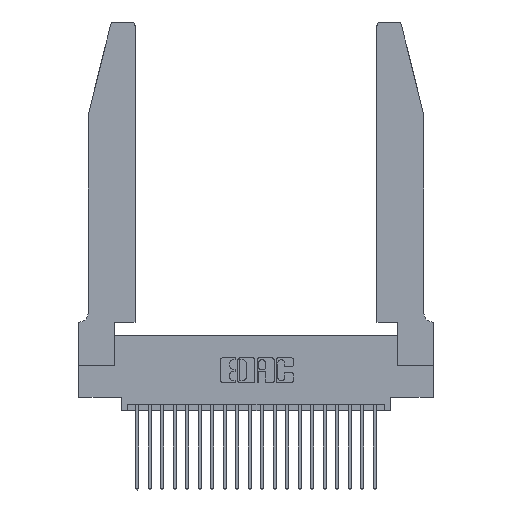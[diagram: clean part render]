
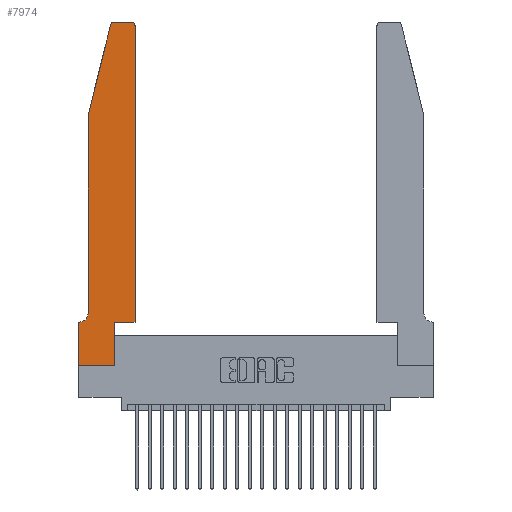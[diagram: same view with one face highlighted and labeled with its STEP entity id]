
A CAD part, top view. The second image highlights one B-rep face of the part: STEP entity #7974.
In plain terms, the highlighted planar face has unit normal (0, 0, 1).
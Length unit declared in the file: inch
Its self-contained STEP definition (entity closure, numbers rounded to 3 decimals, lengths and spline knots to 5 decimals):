
#375 = DIRECTION ( 'NONE',  ( 1., 0., 0. ) ) ;
#386 = EDGE_CURVE ( 'NONE', #14922, #15033, #14284, .T. ) ;
#395 = FACE_OUTER_BOUND ( 'NONE', #5012, .T. ) ;
#712 = DIRECTION ( 'NONE',  ( -1., 0., 0. ) ) ;
#841 = ORIENTED_EDGE ( 'NONE', *, *, #11650, .T. ) ;
#1287 = DIRECTION ( 'NONE',  ( 0., 0., 1. ) ) ;
#1448 = EDGE_CURVE ( 'NONE', #20195, #18270, #11090, .T. ) ;
#1613 = VECTOR ( 'NONE', #18647, 39.37008 ) ;
#2149 = DIRECTION ( 'NONE',  ( -0.239, -0.971, 0. ) ) ;
#2186 = VERTEX_POINT ( 'NONE', #14202 ) ;
#2226 = CARTESIAN_POINT ( 'NONE',  ( 0., 0., 0.37 ) ) ;
#2346 = DIRECTION ( 'NONE',  ( 1., 0., 0. ) ) ;
#2390 = CARTESIAN_POINT ( 'NONE',  ( 0.2865, 0.35, 0.37 ) ) ;
#2464 = EDGE_CURVE ( 'NONE', #11010, #21786, #21974, .T. ) ;
#2804 = CARTESIAN_POINT ( 'NONE',  ( 0., 0., 0.37 ) ) ;
#2820 = CARTESIAN_POINT ( 'NONE',  ( 0.4205, 2.72, 0.37 ) ) ;
#2937 = ORIENTED_EDGE ( 'NONE', *, *, #9304, .T. ) ;
#3006 = CARTESIAN_POINT ( 'NONE',  ( 0.4205, 2.75, 0.37 ) ) ;
#3283 = VECTOR ( 'NONE', #2346, 39.37008 ) ;
#4457 = DIRECTION ( 'NONE',  ( 1., 0., 0. ) ) ;
#4596 = CARTESIAN_POINT ( 'NONE',  ( 0.2605, 2.75, 0.37 ) ) ;
#4702 = CARTESIAN_POINT ( 'NONE',  ( 0., 0., 0.37 ) ) ;
#4712 = CARTESIAN_POINT ( 'NONE',  ( 0.0055, 0.35, 0.37 ) ) ;
#4943 = CARTESIAN_POINT ( 'NONE',  ( 0., 0.35, 0.37 ) ) ;
#4962 = DIRECTION ( 'NONE',  ( 1., 0., 0. ) ) ;
#5012 = EDGE_LOOP ( 'NONE', ( #23389, #8908, #841, #10325, #7568, #16511, #15897, #10751, #23097, #19369, #23200, #2937 ) ) ;
#5309 = LINE ( 'NONE', #2226, #1613 ) ;
#5338 = VERTEX_POINT ( 'NONE', #6586 ) ;
#5339 = VERTEX_POINT ( 'NONE', #4702 ) ;
#6420 = EDGE_CURVE ( 'NONE', #5338, #14922, #22065, .T. ) ;
#6497 = CARTESIAN_POINT ( 'NONE',  ( 0., 0.35, 0.37 ) ) ;
#6501 = CIRCLE ( 'NONE', #16223, 0.03 ) ;
#6586 = CARTESIAN_POINT ( 'NONE',  ( 0.0755, 0.42, 0.37 ) ) ;
#6625 = DIRECTION ( 'NONE',  ( 0., -1., 0. ) ) ;
#7568 = ORIENTED_EDGE ( 'NONE', *, *, #6420, .T. ) ;
#7708 = DIRECTION ( 'NONE',  ( 0., 1., 0. ) ) ;
#7835 = VECTOR ( 'NONE', #7708, 39.37008 ) ;
#7974 = ADVANCED_FACE ( 'NONE', ( #395 ), #19043, .T. ) ;
#8908 = ORIENTED_EDGE ( 'NONE', *, *, #22490, .T. ) ;
#9304 = EDGE_CURVE ( 'NONE', #21786, #20195, #6501, .T. ) ;
#9918 = CARTESIAN_POINT ( 'NONE',  ( 0.0755, 2., 0.37 ) ) ;
#10315 = CARTESIAN_POINT ( 'NONE',  ( 0.0055, 0.42, 0.37 ) ) ;
#10325 = ORIENTED_EDGE ( 'NONE', *, *, #20200, .T. ) ;
#10751 = ORIENTED_EDGE ( 'NONE', *, *, #14930, .T. ) ;
#10755 = CARTESIAN_POINT ( 'NONE',  ( 0.4505, 2.72, 0.37 ) ) ;
#11010 = VERTEX_POINT ( 'NONE', #19975 ) ;
#11090 = LINE ( 'NONE', #4596, #23099 ) ;
#11195 = LINE ( 'NONE', #13364, #3283 ) ;
#11541 = EDGE_CURVE ( 'NONE', #15033, #5339, #5309, .T. ) ;
#11650 = EDGE_CURVE ( 'NONE', #23069, #12090, #20921, .T. ) ;
#12090 = VERTEX_POINT ( 'NONE', #21046 ) ;
#12584 = VECTOR ( 'NONE', #21058, 39.37008 ) ;
#12976 = EDGE_CURVE ( 'NONE', #2186, #11010, #11195, .T. ) ;
#13295 = CARTESIAN_POINT ( 'NONE',  ( 0.4505, 0.35, 0.37 ) ) ;
#13364 = CARTESIAN_POINT ( 'NONE',  ( 0.4505, 0.35, 0.37 ) ) ;
#13487 = CARTESIAN_POINT ( 'NONE',  ( 0.0755, 2., 0.37 ) ) ;
#13875 = DIRECTION ( 'NONE',  ( 0., 0., 1. ) ) ;
#14049 = CARTESIAN_POINT ( 'NONE',  ( 0.0755, 0.35, 0.37 ) ) ;
#14202 = CARTESIAN_POINT ( 'NONE',  ( 0.2865, 0.35, 0.37 ) ) ;
#14284 = LINE ( 'NONE', #14049, #12584 ) ;
#14501 = LINE ( 'NONE', #9918, #22201 ) ;
#14786 = DIRECTION ( 'NONE',  ( 0., 0., -1. ) ) ;
#14827 = DIRECTION ( 'NONE',  ( 0., 0., 1. ) ) ;
#14922 = VERTEX_POINT ( 'NONE', #4712 ) ;
#14930 = EDGE_CURVE ( 'NONE', #5339, #21293, #17022, .T. ) ;
#15033 = VERTEX_POINT ( 'NONE', #4943 ) ;
#15897 = ORIENTED_EDGE ( 'NONE', *, *, #11541, .T. ) ;
#16223 = AXIS2_PLACEMENT_3D ( 'NONE', #2820, #1287, #4962 ) ;
#16422 = CIRCLE ( 'NONE', #21557, 0.03 ) ;
#16439 = AXIS2_PLACEMENT_3D ( 'NONE', #10315, #14786, #712 ) ;
#16511 = ORIENTED_EDGE ( 'NONE', *, *, #386, .T. ) ;
#16526 = CARTESIAN_POINT ( 'NONE',  ( 0.2865, 0., 0.37 ) ) ;
#16674 = EDGE_CURVE ( 'NONE', #21293, #2186, #22053, .T. ) ;
#17022 = LINE ( 'NONE', #2804, #21900 ) ;
#17051 = DIRECTION ( 'NONE',  ( 1., 0., 0. ) ) ;
#17523 = AXIS2_PLACEMENT_3D ( 'NONE', #6497, #13875, #4457 ) ;
#18270 = VERTEX_POINT ( 'NONE', #19004 ) ;
#18383 = CARTESIAN_POINT ( 'NONE',  ( 0.284, 2.72, 0.37 ) ) ;
#18647 = DIRECTION ( 'NONE',  ( 0., -1., 0. ) ) ;
#19004 = CARTESIAN_POINT ( 'NONE',  ( 0.284, 2.75, 0.37 ) ) ;
#19043 = PLANE ( 'NONE',  #17523 ) ;
#19104 = DIRECTION ( 'NONE',  ( -1., 0., 0. ) ) ;
#19369 = ORIENTED_EDGE ( 'NONE', *, *, #12976, .T. ) ;
#19975 = CARTESIAN_POINT ( 'NONE',  ( 0.4505, 0.35, 0.37 ) ) ;
#20195 = VERTEX_POINT ( 'NONE', #3006 ) ;
#20200 = EDGE_CURVE ( 'NONE', #12090, #5338, #14501, .T. ) ;
#20207 = CARTESIAN_POINT ( 'NONE',  ( 0.25487, 2.72718, 0.37 ) ) ;
#20921 = LINE ( 'NONE', #13487, #22674 ) ;
#21046 = CARTESIAN_POINT ( 'NONE',  ( 0.0755, 2., 0.37 ) ) ;
#21058 = DIRECTION ( 'NONE',  ( -1., 0., 0. ) ) ;
#21293 = VERTEX_POINT ( 'NONE', #16526 ) ;
#21557 = AXIS2_PLACEMENT_3D ( 'NONE', #18383, #14827, #375 ) ;
#21786 = VERTEX_POINT ( 'NONE', #10755 ) ;
#21900 = VECTOR ( 'NONE', #17051, 39.37008 ) ;
#21974 = LINE ( 'NONE', #13295, #23151 ) ;
#22053 = LINE ( 'NONE', #2390, #7835 ) ;
#22065 = CIRCLE ( 'NONE', #16439, 0.07 ) ;
#22201 = VECTOR ( 'NONE', #6625, 39.37008 ) ;
#22478 = DIRECTION ( 'NONE',  ( 0., 1., 0. ) ) ;
#22490 = EDGE_CURVE ( 'NONE', #18270, #23069, #16422, .T. ) ;
#22674 = VECTOR ( 'NONE', #2149, 39.37008 ) ;
#23069 = VERTEX_POINT ( 'NONE', #20207 ) ;
#23097 = ORIENTED_EDGE ( 'NONE', *, *, #16674, .T. ) ;
#23099 = VECTOR ( 'NONE', #19104, 39.37008 ) ;
#23151 = VECTOR ( 'NONE', #22478, 39.37008 ) ;
#23200 = ORIENTED_EDGE ( 'NONE', *, *, #2464, .T. ) ;
#23389 = ORIENTED_EDGE ( 'NONE', *, *, #1448, .T. ) ;
